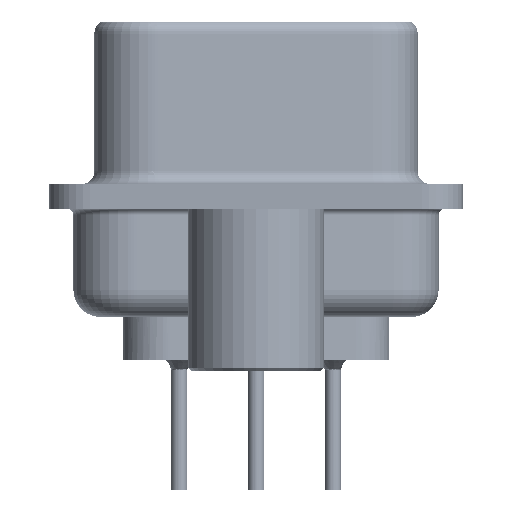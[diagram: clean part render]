
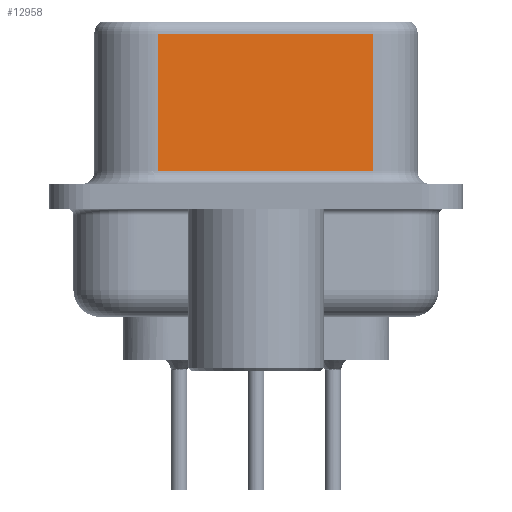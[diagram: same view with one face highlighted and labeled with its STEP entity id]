
A CAD part, left-side view. The second image highlights one B-rep face of the part: STEP entity #12958.
In plain terms, the highlighted planar face has unit normal (-0.985, -0.174, 0).
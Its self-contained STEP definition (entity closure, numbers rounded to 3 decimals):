
#277 = VECTOR ( 'NONE', #6253, 1000. ) ;
#2148 = VECTOR ( 'NONE', #25531, 1000. ) ;
#3006 = ORIENTED_EDGE ( 'NONE', *, *, #12008, .T. ) ;
#4646 = CARTESIAN_POINT ( 'NONE',  ( 5.132, -4.322, 6.02 ) ) ;
#5590 = DIRECTION ( 'NONE',  ( 0.985, 0.174, 0. ) ) ;
#5742 = ORIENTED_EDGE ( 'NONE', *, *, #30483, .T. ) ;
#6253 = DIRECTION ( 'NONE',  ( -0.174, 0.985, 0. ) ) ;
#7601 = LINE ( 'NONE', #29854, #2148 ) ;
#7825 = EDGE_LOOP ( 'NONE', ( #18986, #5742, #3006, #29504 ) ) ;
#7838 = CARTESIAN_POINT ( 'NONE',  ( 3.73, 3.628, 6.02 ) ) ;
#8659 = AXIS2_PLACEMENT_3D ( 'NONE', #8737, #5590, #28580 ) ;
#8737 = CARTESIAN_POINT ( 'NONE',  ( 5.132, -4.322, 6.52 ) ) ;
#9609 = DIRECTION ( 'NONE',  ( 0., 0., -1. ) ) ;
#11926 = EDGE_CURVE ( 'NONE', #17068, #13215, #7601, .T. ) ;
#12008 = EDGE_CURVE ( 'NONE', #12877, #17068, #21695, .T. ) ;
#12877 = VERTEX_POINT ( 'NONE', #7838 ) ;
#12958 = ADVANCED_FACE ( 'NONE', ( #14134 ), #20238, .F. ) ;
#13215 = VERTEX_POINT ( 'NONE', #35400 ) ;
#13536 = EDGE_CURVE ( 'NONE', #21426, #13215, #23708, .T. ) ;
#14134 = FACE_OUTER_BOUND ( 'NONE', #7825, .T. ) ;
#17068 = VERTEX_POINT ( 'NONE', #35482 ) ;
#17541 = VECTOR ( 'NONE', #9609, 1000. ) ;
#18986 = ORIENTED_EDGE ( 'NONE', *, *, #13536, .F. ) ;
#20238 = PLANE ( 'NONE',  #8659 ) ;
#21095 = CARTESIAN_POINT ( 'NONE',  ( 5.132, -4.322, 6.52 ) ) ;
#21426 = VERTEX_POINT ( 'NONE', #4646 ) ;
#21695 = LINE ( 'NONE', #24660, #28791 ) ;
#23708 = LINE ( 'NONE', #21095, #17541 ) ;
#24660 = CARTESIAN_POINT ( 'NONE',  ( 3.73, 3.628, 6.52 ) ) ;
#25531 = DIRECTION ( 'NONE',  ( 0.174, -0.985, 0. ) ) ;
#28580 = DIRECTION ( 'NONE',  ( -0.174, 0.985, 0. ) ) ;
#28791 = VECTOR ( 'NONE', #35948, 1000. ) ;
#28883 = CARTESIAN_POINT ( 'NONE',  ( 5.132, -4.322, 6.02 ) ) ;
#29504 = ORIENTED_EDGE ( 'NONE', *, *, #11926, .T. ) ;
#29854 = CARTESIAN_POINT ( 'NONE',  ( 5.132, -4.322, 0.95 ) ) ;
#30483 = EDGE_CURVE ( 'NONE', #21426, #12877, #34794, .T. ) ;
#34794 = LINE ( 'NONE', #28883, #277 ) ;
#35400 = CARTESIAN_POINT ( 'NONE',  ( 5.132, -4.322, 0.95 ) ) ;
#35482 = CARTESIAN_POINT ( 'NONE',  ( 3.73, 3.628, 0.95 ) ) ;
#35948 = DIRECTION ( 'NONE',  ( 0., 0., -1. ) ) ;
